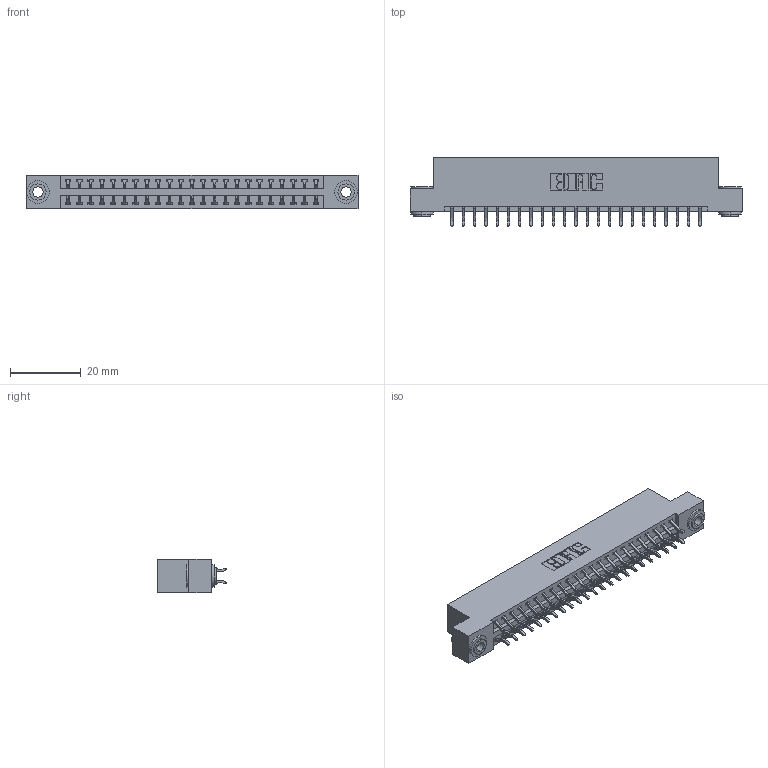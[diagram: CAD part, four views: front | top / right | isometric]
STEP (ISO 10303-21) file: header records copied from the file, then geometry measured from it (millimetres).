
FILE_DESCRIPTION (( 'STEP AP203' ), '1' );
FILE_NAME ('346-046-556-203.STEP', '2022-05-20T20:19:51', ( '' ), ( '' ), 'SwSTEP 2.0', 'SolidWorks 2020', '' );
FILE_SCHEMA (( 'CONFIG_CONTROL_DESIGN' ));
Length unit declared in the file: inch
Products named in the file (4): 345-250-002_345-250-002-102; 346 Part_Flush Mounting Lugs - 0.156 Dia-TH; 345-292-001_556 Tail; 346-046-556-203
Assembly tree (49 placements, depth 2):
  346-046-556-203
    346 Part_Flush Mounting Lugs - 0.156 Dia-TH
    345-292-001_556 Tail  x46
    345-250-002_345-250-002-102  x2
Bounding box: 93.6 x 19.57 x 9.4 mm (x, y, z)
Volume: 8979 mm3; surface area: 12249.6 mm2
Topology: 49 solids, 49 shells, 2842 faces, 8399 edges, 5534 vertices
Faces by surface type: plane 1894, cylinder 940, cone 8
Entity records: 18854 total; most frequent: CARTESIAN_POINT 3129, ORIENTED_EDGE 3042, DIRECTION 2827, EDGE_CURVE 1521, LINE 1265, VECTOR 1265, VERTEX_POINT 1010, AXIS2_PLACEMENT_3D 781
